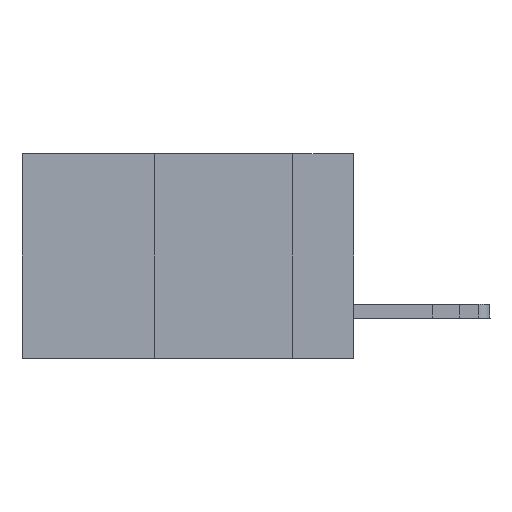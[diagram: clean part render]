
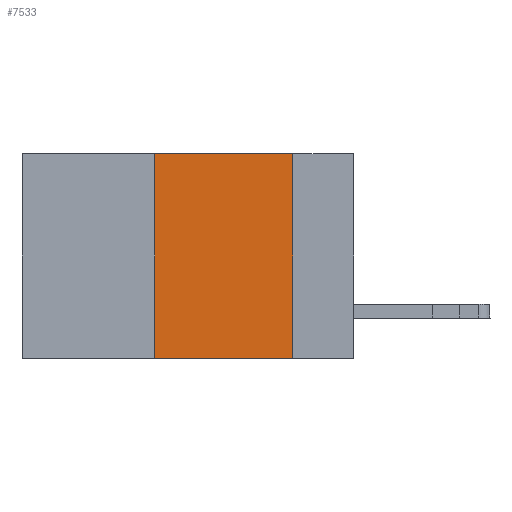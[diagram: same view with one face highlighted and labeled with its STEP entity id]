
A CAD part, left-side view. The second image highlights one B-rep face of the part: STEP entity #7533.
In plain terms, the highlighted planar face has unit normal (-1, 0, 0).
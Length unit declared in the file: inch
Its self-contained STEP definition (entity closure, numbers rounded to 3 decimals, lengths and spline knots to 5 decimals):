
#491 = VECTOR ( 'NONE', #16629, 39.37008 ) ;
#1116 = VERTEX_POINT ( 'NONE', #12980 ) ;
#1184 = LINE ( 'NONE', #8448, #16243 ) ;
#2024 = VECTOR ( 'NONE', #5850, 39.37008 ) ;
#2176 = ORIENTED_EDGE ( 'NONE', *, *, #16588, .T. ) ;
#2663 = LINE ( 'NONE', #13201, #2024 ) ;
#4289 = EDGE_CURVE ( 'NONE', #1116, #22290, #1184, .T. ) ;
#5850 = DIRECTION ( 'NONE',  ( 0., 0., 1. ) ) ;
#7260 = ORIENTED_EDGE ( 'NONE', *, *, #4289, .F. ) ;
#7478 = ORIENTED_EDGE ( 'NONE', *, *, #8667, .F. ) ;
#7485 = EDGE_CURVE ( 'NONE', #21173, #13938, #2663, .T. ) ;
#7533 = ADVANCED_FACE ( 'NONE', ( #15338 ), #13348, .F. ) ;
#7765 = DIRECTION ( 'NONE',  ( 0., 0., -1. ) ) ;
#7903 = DIRECTION ( 'NONE',  ( 1., 0., 0. ) ) ;
#8448 = CARTESIAN_POINT ( 'NONE',  ( 0., 0.11, 0. ) ) ;
#8605 = CARTESIAN_POINT ( 'NONE',  ( 0., 0.36, 0. ) ) ;
#8667 = EDGE_CURVE ( 'NONE', #13938, #1116, #15320, .T. ) ;
#8782 = LINE ( 'NONE', #17160, #17400 ) ;
#9313 = CARTESIAN_POINT ( 'NONE',  ( 0., 0.36, -0.37 ) ) ;
#11553 = ORIENTED_EDGE ( 'NONE', *, *, #7485, .F. ) ;
#11693 = DIRECTION ( 'NONE',  ( 0., -1., 0. ) ) ;
#12980 = CARTESIAN_POINT ( 'NONE',  ( 0., 0.11, 0. ) ) ;
#13201 = CARTESIAN_POINT ( 'NONE',  ( 0., 0.36, 0. ) ) ;
#13348 = PLANE ( 'NONE',  #19891 ) ;
#13938 = VERTEX_POINT ( 'NONE', #8605 ) ;
#14766 = CARTESIAN_POINT ( 'NONE',  ( 0., 0.6, 0. ) ) ;
#15320 = LINE ( 'NONE', #14766, #491 ) ;
#15338 = FACE_OUTER_BOUND ( 'NONE', #18304, .T. ) ;
#16243 = VECTOR ( 'NONE', #7765, 39.37008 ) ;
#16588 = EDGE_CURVE ( 'NONE', #21173, #22290, #8782, .T. ) ;
#16629 = DIRECTION ( 'NONE',  ( 0., -1., 0. ) ) ;
#17160 = CARTESIAN_POINT ( 'NONE',  ( 0., 0.6, -0.37 ) ) ;
#17400 = VECTOR ( 'NONE', #11693, 39.37008 ) ;
#18304 = EDGE_LOOP ( 'NONE', ( #7260, #7478, #11553, #2176 ) ) ;
#18912 = CARTESIAN_POINT ( 'NONE',  ( 0., 0.6, 0. ) ) ;
#19891 = AXIS2_PLACEMENT_3D ( 'NONE', #18912, #7903, #20778 ) ;
#20778 = DIRECTION ( 'NONE',  ( 0., 0., -1. ) ) ;
#21173 = VERTEX_POINT ( 'NONE', #9313 ) ;
#22290 = VERTEX_POINT ( 'NONE', #23809 ) ;
#23809 = CARTESIAN_POINT ( 'NONE',  ( 0., 0.11, -0.37 ) ) ;
